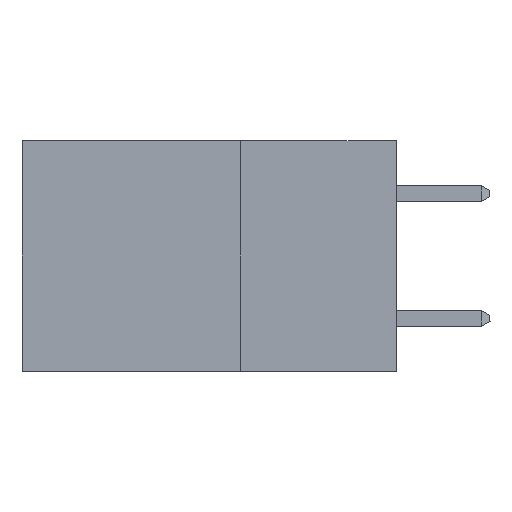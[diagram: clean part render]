
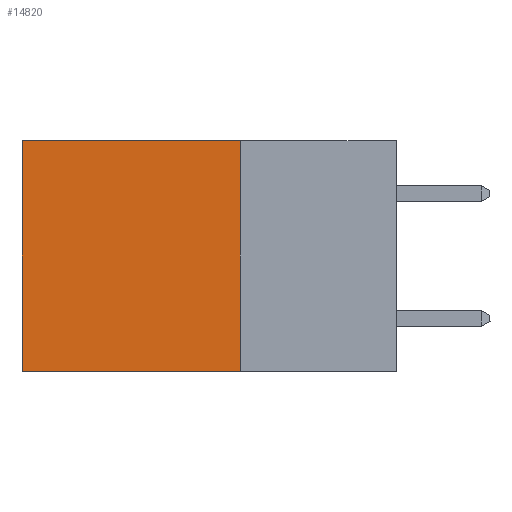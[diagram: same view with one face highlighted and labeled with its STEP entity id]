
A CAD part, left-side view. The second image highlights one B-rep face of the part: STEP entity #14820.
In plain terms, the highlighted planar face has unit normal (-1, 0, 0).
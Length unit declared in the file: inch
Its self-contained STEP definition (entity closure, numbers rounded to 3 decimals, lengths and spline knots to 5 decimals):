
#243 = ORIENTED_EDGE ( 'NONE', *, *, #16159, .T. ) ;
#1335 = EDGE_CURVE ( 'NONE', #17433, #26348, #3820, .T. ) ;
#3160 = CARTESIAN_POINT ( 'NONE',  ( 0.298, 0.6, 0. ) ) ;
#3676 = EDGE_CURVE ( 'NONE', #27344, #26348, #7647, .T. ) ;
#3820 = LINE ( 'NONE', #16249, #17375 ) ;
#7647 = LINE ( 'NONE', #19974, #17914 ) ;
#7688 = LINE ( 'NONE', #22059, #18566 ) ;
#8542 = LINE ( 'NONE', #23781, #27432 ) ;
#9394 = DIRECTION ( 'NONE',  ( 0., 1., 0. ) ) ;
#10296 = ORIENTED_EDGE ( 'NONE', *, *, #25139, .F. ) ;
#10900 = CARTESIAN_POINT ( 'NONE',  ( 0.298, 0.25, -0.37 ) ) ;
#13223 = DIRECTION ( 'NONE',  ( 1., 0., 0. ) ) ;
#13332 = VERTEX_POINT ( 'NONE', #22928 ) ;
#14306 = ORIENTED_EDGE ( 'NONE', *, *, #3676, .T. ) ;
#14820 = ADVANCED_FACE ( 'NONE', ( #16356 ), #21525, .F. ) ;
#14845 = ORIENTED_EDGE ( 'NONE', *, *, #1335, .F. ) ;
#15651 = DIRECTION ( 'NONE',  ( 0., 0., -1. ) ) ;
#16159 = EDGE_CURVE ( 'NONE', #13332, #27344, #7688, .T. ) ;
#16249 = CARTESIAN_POINT ( 'NONE',  ( 0.298, 0.25, -0.37 ) ) ;
#16356 = FACE_OUTER_BOUND ( 'NONE', #24881, .T. ) ;
#17196 = DIRECTION ( 'NONE',  ( 0., 0., -1. ) ) ;
#17375 = VECTOR ( 'NONE', #20210, 39.37008 ) ;
#17433 = VERTEX_POINT ( 'NONE', #10900 ) ;
#17914 = VECTOR ( 'NONE', #15651, 39.37008 ) ;
#18566 = VECTOR ( 'NONE', #9394, 39.37008 ) ;
#19974 = CARTESIAN_POINT ( 'NONE',  ( 0.298, 0.6, 0. ) ) ;
#20210 = DIRECTION ( 'NONE',  ( 0., 1., 0. ) ) ;
#21525 = PLANE ( 'NONE',  #25728 ) ;
#21954 = DIRECTION ( 'NONE',  ( 0., 0., -1. ) ) ;
#22059 = CARTESIAN_POINT ( 'NONE',  ( 0.298, 0.25, 0. ) ) ;
#22928 = CARTESIAN_POINT ( 'NONE',  ( 0.298, 0.25, 0. ) ) ;
#23781 = CARTESIAN_POINT ( 'NONE',  ( 0.298, 0.25, 0. ) ) ;
#24202 = CARTESIAN_POINT ( 'NONE',  ( 0.298, 0.6, -0.37 ) ) ;
#24881 = EDGE_LOOP ( 'NONE', ( #14306, #14845, #10296, #243 ) ) ;
#25139 = EDGE_CURVE ( 'NONE', #13332, #17433, #8542, .T. ) ;
#25728 = AXIS2_PLACEMENT_3D ( 'NONE', #25964, #13223, #17196 ) ;
#25964 = CARTESIAN_POINT ( 'NONE',  ( 0.298, 0.25, 0. ) ) ;
#26348 = VERTEX_POINT ( 'NONE', #24202 ) ;
#27344 = VERTEX_POINT ( 'NONE', #3160 ) ;
#27432 = VECTOR ( 'NONE', #21954, 39.37008 ) ;
